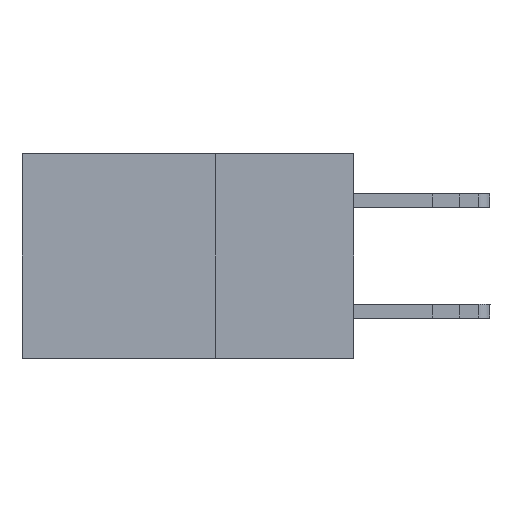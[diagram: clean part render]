
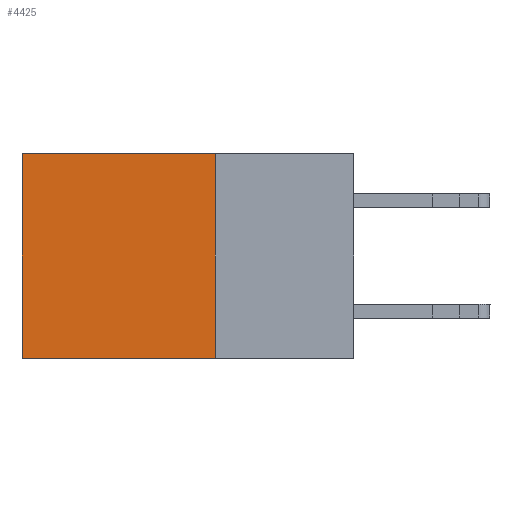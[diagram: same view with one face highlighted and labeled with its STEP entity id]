
A CAD part, left-side view. The second image highlights one B-rep face of the part: STEP entity #4425.
In plain terms, the highlighted planar face has unit normal (-1, 0, 0).
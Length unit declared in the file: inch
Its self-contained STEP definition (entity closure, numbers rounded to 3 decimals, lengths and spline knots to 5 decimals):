
#16 = VECTOR ( 'NONE', #4541, 39.37008 ) ;
#65 = EDGE_CURVE ( 'NONE', #15492, #13290, #8757, .T. ) ;
#71 = LINE ( 'NONE', #9221, #16 ) ;
#883 = DIRECTION ( 'NONE',  ( 1., 0., 0. ) ) ;
#1362 = LINE ( 'NONE', #8698, #9364 ) ;
#2381 = CARTESIAN_POINT ( 'NONE',  ( 0.2875, 0.6, -0.37 ) ) ;
#2410 = DIRECTION ( 'NONE',  ( 0., 0., -1. ) ) ;
#2509 = PLANE ( 'NONE',  #6552 ) ;
#2702 = ORIENTED_EDGE ( 'NONE', *, *, #9397, .F. ) ;
#3507 = VERTEX_POINT ( 'NONE', #16248 ) ;
#3864 = FACE_OUTER_BOUND ( 'NONE', #5240, .T. ) ;
#3991 = DIRECTION ( 'NONE',  ( 0., 0., -1. ) ) ;
#4085 = LINE ( 'NONE', #4176, #10658 ) ;
#4176 = CARTESIAN_POINT ( 'NONE',  ( 0.2875, 0.25, 0. ) ) ;
#4201 = EDGE_CURVE ( 'NONE', #18886, #3507, #4085, .T. ) ;
#4425 = ADVANCED_FACE ( 'NONE', ( #3864 ), #2509, .F. ) ;
#4541 = DIRECTION ( 'NONE',  ( 0., 1., 0. ) ) ;
#5240 = EDGE_LOOP ( 'NONE', ( #18914, #2702, #17841, #18741 ) ) ;
#5690 = CARTESIAN_POINT ( 'NONE',  ( 0.2875, 0.6, 0. ) ) ;
#6552 = AXIS2_PLACEMENT_3D ( 'NONE', #10032, #883, #2410 ) ;
#7434 = CARTESIAN_POINT ( 'NONE',  ( 0.2875, 0.6, 0. ) ) ;
#8698 = CARTESIAN_POINT ( 'NONE',  ( 0.2875, 0.25, -0.37 ) ) ;
#8757 = LINE ( 'NONE', #5690, #9550 ) ;
#9221 = CARTESIAN_POINT ( 'NONE',  ( 0.2875, 0.25, 0. ) ) ;
#9364 = VECTOR ( 'NONE', #17879, 39.37008 ) ;
#9397 = EDGE_CURVE ( 'NONE', #3507, #13290, #1362, .T. ) ;
#9550 = VECTOR ( 'NONE', #19432, 39.37008 ) ;
#10032 = CARTESIAN_POINT ( 'NONE',  ( 0.2875, 0.25, 0. ) ) ;
#10658 = VECTOR ( 'NONE', #3991, 39.37008 ) ;
#13290 = VERTEX_POINT ( 'NONE', #2381 ) ;
#14106 = CARTESIAN_POINT ( 'NONE',  ( 0.2875, 0.25, 0. ) ) ;
#15492 = VERTEX_POINT ( 'NONE', #7434 ) ;
#15709 = EDGE_CURVE ( 'NONE', #18886, #15492, #71, .T. ) ;
#16248 = CARTESIAN_POINT ( 'NONE',  ( 0.2875, 0.25, -0.37 ) ) ;
#17841 = ORIENTED_EDGE ( 'NONE', *, *, #4201, .F. ) ;
#17879 = DIRECTION ( 'NONE',  ( 0., 1., 0. ) ) ;
#18741 = ORIENTED_EDGE ( 'NONE', *, *, #15709, .T. ) ;
#18886 = VERTEX_POINT ( 'NONE', #14106 ) ;
#18914 = ORIENTED_EDGE ( 'NONE', *, *, #65, .T. ) ;
#19432 = DIRECTION ( 'NONE',  ( 0., 0., -1. ) ) ;
